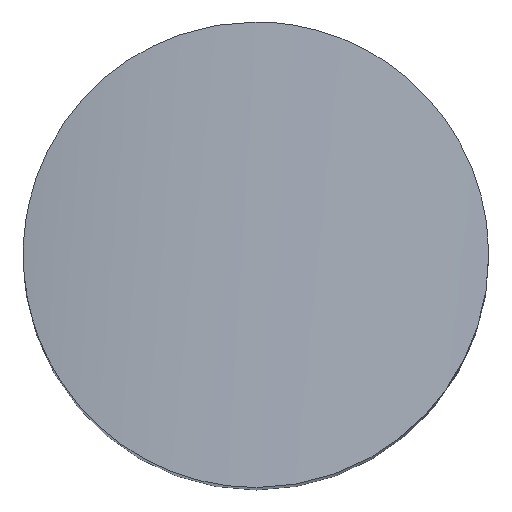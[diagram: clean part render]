
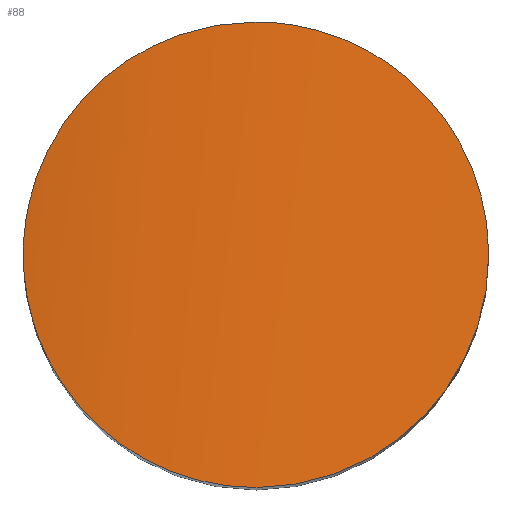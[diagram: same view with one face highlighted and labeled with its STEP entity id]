
A CAD part, top view. The second image highlights one B-rep face of the part: STEP entity #88.
In plain terms, the highlighted cylindrical face has radius 10 mm (diameter 20 mm), a partial arc.
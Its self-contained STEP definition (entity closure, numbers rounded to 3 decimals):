
#5 = CARTESIAN_POINT ( 'NONE',  ( 2.498, 8.937, 5.441 ) ) ;
#14 = CYLINDRICAL_SURFACE ( 'NONE', #178, 10. ) ;
#23 = FACE_OUTER_BOUND ( 'NONE', #26, .T. ) ;
#26 = EDGE_LOOP ( 'NONE', ( #60, #62 ) ) ;
#30 = VERTEX_POINT ( 'NONE', #126 ) ;
#40 = VERTEX_POINT ( 'NONE', #186 ) ;
#44 = CARTESIAN_POINT ( 'NONE',  ( -1.053, 11.008, 7.312 ) ) ;
#47 = B_SPLINE_CURVE_WITH_KNOTS ( 'NONE', 3,
 ( #119, #173, #112, #113, #115, #131, #122, #139, #136, #143, #140, #142, #148, #145, #144, #5, #163, #138, #156, #155, #154, #147, #132, #134, #161, #100, #105, #102, #97, #104 ),
 .UNSPECIFIED., .F., .F.,
 ( 4, 2, 2, 2, 2, 2, 2, 2, 2, 2, 2, 2, 2, 2, 4 ),
 ( 0., 0.001, 0.001, 0.002, 0.002, 0.003, 0.003, 0.004, 0.005, 0.005, 0.006, 0.006, 0.007, 0.007, 0.008 ),
 .UNSPECIFIED. ) ;
#57 = EDGE_CURVE ( 'NONE', #40, #30, #73, .T. ) ;
#58 = EDGE_CURVE ( 'NONE', #30, #40, #47, .T. ) ;
#60 = ORIENTED_EDGE ( 'NONE', *, *, #57, .T. ) ;
#62 = ORIENTED_EDGE ( 'NONE', *, *, #58, .T. ) ;
#67 = CARTESIAN_POINT ( 'NONE',  ( 0., 11.235, 6.591 ) ) ;
#68 = CARTESIAN_POINT ( 'NONE',  ( -2.111, 7.386, 7.951 ) ) ;
#69 = CARTESIAN_POINT ( 'NONE',  ( -2.474, 8.335, 8.418 ) ) ;
#71 = CARTESIAN_POINT ( 'NONE',  ( -1.821, 7.015, 7.65 ) ) ;
#72 = CARTESIAN_POINT ( 'NONE',  ( -1.597, 6.805, 7.441 ) ) ;
#73 = B_SPLINE_CURVE_WITH_KNOTS ( 'NONE', 3,
 ( #67, #137, #103, #44, #181, #150, #124, #123, #125, #127, #160, #129, #135, #79, #69, #108, #158, #84, #68, #106, #71, #72, #74, #76, #78, #89, #90, #92, #107, #111 ),
 .UNSPECIFIED., .F., .F.,
 ( 4, 2, 2, 2, 2, 2, 2, 2, 2, 2, 2, 2, 2, 2, 4 ),
 ( 0.008, 0.009, 0.01, 0.01, 0.012, 0.012, 0.013, 0.013, 0.014, 0.014, 0.015, 0.015, 0.016, 0.017, 0.017 ),
 .UNSPECIFIED. ) ;
#74 = CARTESIAN_POINT ( 'NONE',  ( -1.474, 6.71, 7.333 ) ) ;
#76 = CARTESIAN_POINT ( 'NONE',  ( -1.215, 6.545, 7.12 ) ) ;
#78 = CARTESIAN_POINT ( 'NONE',  ( -1.079, 6.474, 7.015 ) ) ;
#79 = CARTESIAN_POINT ( 'NONE',  ( -2.497, 8.517, 8.463 ) ) ;
#82 = CARTESIAN_POINT ( 'NONE',  ( 5.666, 15.746, 15.115 ) ) ;
#84 = CARTESIAN_POINT ( 'NONE',  ( -2.195, 7.527, 8.047 ) ) ;
#88 = ADVANCED_FACE ( 'NONE', ( #23 ), #14, .F. ) ;
#89 = CARTESIAN_POINT ( 'NONE',  ( -0.792, 6.359, 6.809 ) ) ;
#90 = CARTESIAN_POINT ( 'NONE',  ( -0.64, 6.313, 6.706 ) ) ;
#92 = CARTESIAN_POINT ( 'NONE',  ( -0.327, 6.251, 6.51 ) ) ;
#97 = CARTESIAN_POINT ( 'NONE',  ( 0.295, 11.235, 6.411 ) ) ;
#100 = CARTESIAN_POINT ( 'NONE',  ( 1.175, 10.947, 5.963 ) ) ;
#101 = DIRECTION ( 'NONE',  ( 0.092, 0.996, 0. ) ) ;
#102 = CARTESIAN_POINT ( 'NONE',  ( 0.597, 11.182, 6.245 ) ) ;
#103 = CARTESIAN_POINT ( 'NONE',  ( -0.624, 11.175, 6.993 ) ) ;
#104 = CARTESIAN_POINT ( 'NONE',  ( 0., 11.235, 6.591 ) ) ;
#105 = CARTESIAN_POINT ( 'NONE',  ( 1.031, 11.018, 6.03 ) ) ;
#106 = CARTESIAN_POINT ( 'NONE',  ( -1.924, 7.131, 7.753 ) ) ;
#107 = CARTESIAN_POINT ( 'NONE',  ( -0.166, 6.235, 6.416 ) ) ;
#108 = CARTESIAN_POINT ( 'NONE',  ( -2.392, 7.988, 8.295 ) ) ;
#111 = CARTESIAN_POINT ( 'NONE',  ( 0., 6.235, 6.327 ) ) ;
#112 = CARTESIAN_POINT ( 'NONE',  ( 0.304, 6.249, 6.168 ) ) ;
#113 = CARTESIAN_POINT ( 'NONE',  ( 0.608, 6.305, 6.025 ) ) ;
#115 = CARTESIAN_POINT ( 'NONE',  ( 0.762, 6.348, 5.959 ) ) ;
#119 = CARTESIAN_POINT ( 'NONE',  ( 0., 6.235, 6.327 ) ) ;
#122 = CARTESIAN_POINT ( 'NONE',  ( 1.205, 6.538, 5.784 ) ) ;
#123 = CARTESIAN_POINT ( 'NONE',  ( -1.923, 10.363, 8.031 ) ) ;
#124 = CARTESIAN_POINT ( 'NONE',  ( -1.575, 10.683, 7.732 ) ) ;
#125 = CARTESIAN_POINT ( 'NONE',  ( -2.127, 10.096, 8.217 ) ) ;
#126 = CARTESIAN_POINT ( 'NONE',  ( 0., 6.235, 6.327 ) ) ;
#127 = CARTESIAN_POINT ( 'NONE',  ( -2.347, 9.614, 8.408 ) ) ;
#128 = DIRECTION ( 'NONE',  ( -0.996, 0.092, 0. ) ) ;
#129 = CARTESIAN_POINT ( 'NONE',  ( -2.484, 9.076, 8.506 ) ) ;
#131 = CARTESIAN_POINT ( 'NONE',  ( 1.061, 6.466, 5.838 ) ) ;
#132 = CARTESIAN_POINT ( 'NONE',  ( 1.819, 10.458, 5.691 ) ) ;
#134 = CARTESIAN_POINT ( 'NONE',  ( 1.578, 10.681, 5.787 ) ) ;
#135 = CARTESIAN_POINT ( 'NONE',  ( -2.502, 8.891, 8.507 ) ) ;
#136 = CARTESIAN_POINT ( 'NONE',  ( 1.614, 6.818, 5.646 ) ) ;
#137 = CARTESIAN_POINT ( 'NONE',  ( -0.321, 11.235, 6.787 ) ) ;
#138 = CARTESIAN_POINT ( 'NONE',  ( 2.404, 9.442, 5.478 ) ) ;
#139 = CARTESIAN_POINT ( 'NONE',  ( 1.481, 6.714, 5.688 ) ) ;
#140 = CARTESIAN_POINT ( 'NONE',  ( 1.963, 7.178, 5.545 ) ) ;
#142 = CARTESIAN_POINT ( 'NONE',  ( 2.156, 7.457, 5.496 ) ) ;
#143 = CARTESIAN_POINT ( 'NONE',  ( 1.855, 7.05, 5.575 ) ) ;
#144 = CARTESIAN_POINT ( 'NONE',  ( 2.504, 8.424, 5.427 ) ) ;
#145 = CARTESIAN_POINT ( 'NONE',  ( 2.436, 8.079, 5.436 ) ) ;
#147 = CARTESIAN_POINT ( 'NONE',  ( 1.931, 10.332, 5.648 ) ) ;
#148 = CARTESIAN_POINT ( 'NONE',  ( 2.239, 7.609, 5.477 ) ) ;
#150 = CARTESIAN_POINT ( 'NONE',  ( -1.452, 10.776, 7.629 ) ) ;
#154 = CARTESIAN_POINT ( 'NONE',  ( 2.126, 10.061, 5.576 ) ) ;
#155 = CARTESIAN_POINT ( 'NONE',  ( 2.211, 9.914, 5.546 ) ) ;
#156 = CARTESIAN_POINT ( 'NONE',  ( 2.351, 9.603, 5.497 ) ) ;
#158 = CARTESIAN_POINT ( 'NONE',  ( -2.335, 7.827, 8.218 ) ) ;
#160 = CARTESIAN_POINT ( 'NONE',  ( -2.405, 9.442, 8.455 ) ) ;
#161 = CARTESIAN_POINT ( 'NONE',  ( 1.448, 10.779, 5.841 ) ) ;
#163 = CARTESIAN_POINT ( 'NONE',  ( 2.478, 9.11, 5.45 ) ) ;
#173 = CARTESIAN_POINT ( 'NONE',  ( 0.152, 6.235, 6.245 ) ) ;
#178 = AXIS2_PLACEMENT_3D ( 'NONE', #82, #101, #128 ) ;
#181 = CARTESIAN_POINT ( 'NONE',  ( -1.191, 10.938, 7.42 ) ) ;
#186 = CARTESIAN_POINT ( 'NONE',  ( 0., 11.235, 6.591 ) ) ;
